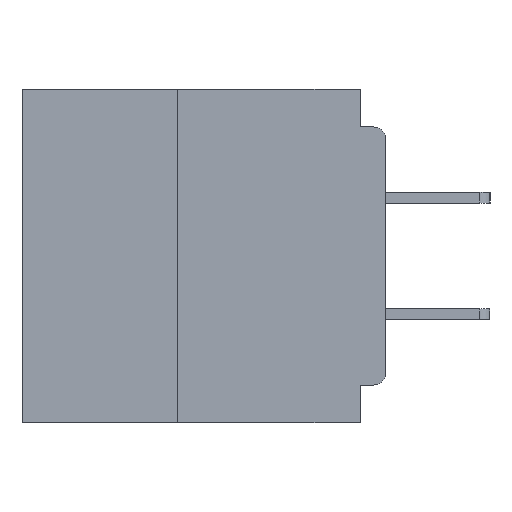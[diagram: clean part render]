
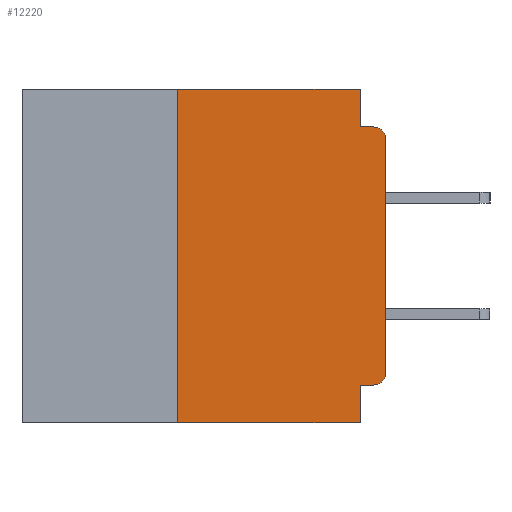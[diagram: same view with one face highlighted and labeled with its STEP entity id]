
A CAD part, left-side view. The second image highlights one B-rep face of the part: STEP entity #12220.
In plain terms, the highlighted planar face has unit normal (-1, 0, 0).
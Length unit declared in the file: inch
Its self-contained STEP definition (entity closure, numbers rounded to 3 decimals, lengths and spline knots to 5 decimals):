
#290 = EDGE_CURVE ( 'NONE', #17240, #39688, #41351, .T. ) ;
#2106 = VECTOR ( 'NONE', #35604, 39.37008 ) ;
#2273 = AXIS2_PLACEMENT_3D ( 'NONE', #43329, #23393, #3260 ) ;
#3179 = LINE ( 'NONE', #18745, #2106 ) ;
#3260 = DIRECTION ( 'NONE',  ( 0., 0., -1. ) ) ;
#4384 = ORIENTED_EDGE ( 'NONE', *, *, #42778, .F. ) ;
#4550 = EDGE_CURVE ( 'NONE', #42149, #12079, #9483, .T. ) ;
#6337 = VECTOR ( 'NONE', #36589, 39.37008 ) ;
#6389 = DIRECTION ( 'NONE',  ( 0., 0., -1. ) ) ;
#6859 = CARTESIAN_POINT ( 'NONE',  ( 0., 0., -0.06 ) ) ;
#7422 = ORIENTED_EDGE ( 'NONE', *, *, #15491, .F. ) ;
#8079 = LINE ( 'NONE', #9819, #24924 ) ;
#9199 = CIRCLE ( 'NONE', #23481, 0.015 ) ;
#9483 = LINE ( 'NONE', #37488, #17401 ) ;
#9774 = CARTESIAN_POINT ( 'NONE',  ( 0., 0.031, -0.4 ) ) ;
#9819 = CARTESIAN_POINT ( 'NONE',  ( 0., 0.031, 0. ) ) ;
#10661 = DIRECTION ( 'NONE',  ( 0., 1., 0. ) ) ;
#11162 = LINE ( 'NONE', #37138, #19002 ) ;
#11334 = PLANE ( 'NONE',  #36453 ) ;
#11867 = CARTESIAN_POINT ( 'NONE',  ( 0., 0., -0.34 ) ) ;
#12079 = VERTEX_POINT ( 'NONE', #40723 ) ;
#12220 = ADVANCED_FACE ( 'NONE', ( #42711 ), #11334, .F. ) ;
#13265 = CARTESIAN_POINT ( 'NONE',  ( 0., 0.015, -0.34 ) ) ;
#14462 = VECTOR ( 'NONE', #22229, 39.37008 ) ;
#14726 = DIRECTION ( 'NONE',  ( 1., 0., 0. ) ) ;
#15491 = EDGE_CURVE ( 'NONE', #17240, #26079, #11162, .T. ) ;
#15524 = CARTESIAN_POINT ( 'NONE',  ( 0., 0., 0. ) ) ;
#16160 = ORIENTED_EDGE ( 'NONE', *, *, #29228, .T. ) ;
#16396 = EDGE_CURVE ( 'NONE', #26079, #41114, #3179, .T. ) ;
#16649 = DIRECTION ( 'NONE',  ( 0., 0., -1. ) ) ;
#16746 = DIRECTION ( 'NONE',  ( 0., 0., -1. ) ) ;
#17018 = VERTEX_POINT ( 'NONE', #39463 ) ;
#17073 = DIRECTION ( 'NONE',  ( 0., 0., 1. ) ) ;
#17240 = VERTEX_POINT ( 'NONE', #27374 ) ;
#17401 = VECTOR ( 'NONE', #10661, 39.37008 ) ;
#18265 = ORIENTED_EDGE ( 'NONE', *, *, #35848, .T. ) ;
#18745 = CARTESIAN_POINT ( 'NONE',  ( 0., 0.437, 0. ) ) ;
#18962 = ORIENTED_EDGE ( 'NONE', *, *, #16396, .F. ) ;
#19002 = VECTOR ( 'NONE', #17073, 39.37008 ) ;
#19512 = ORIENTED_EDGE ( 'NONE', *, *, #290, .T. ) ;
#19656 = CARTESIAN_POINT ( 'NONE',  ( 0., 0.015, -0.355 ) ) ;
#20875 = CARTESIAN_POINT ( 'NONE',  ( 0., 0.25, 0. ) ) ;
#21302 = CARTESIAN_POINT ( 'NONE',  ( 0., 0.437, 0. ) ) ;
#22229 = DIRECTION ( 'NONE',  ( 0., 0., 1. ) ) ;
#23393 = DIRECTION ( 'NONE',  ( -1., 0., 0. ) ) ;
#23481 = AXIS2_PLACEMENT_3D ( 'NONE', #13265, #36714, #16649 ) ;
#24924 = VECTOR ( 'NONE', #16746, 39.37008 ) ;
#25423 = LINE ( 'NONE', #9774, #42065 ) ;
#25580 = DIRECTION ( 'NONE',  ( 0., -1., 0. ) ) ;
#25952 = CARTESIAN_POINT ( 'NONE',  ( 0., 0.015, -0.045 ) ) ;
#25984 = ORIENTED_EDGE ( 'NONE', *, *, #27196, .F. ) ;
#26079 = VERTEX_POINT ( 'NONE', #20875 ) ;
#26563 = CARTESIAN_POINT ( 'NONE',  ( 0., 0.437, -0.4 ) ) ;
#27087 = VERTEX_POINT ( 'NONE', #25952 ) ;
#27196 = EDGE_CURVE ( 'NONE', #12079, #39688, #25423, .T. ) ;
#27374 = CARTESIAN_POINT ( 'NONE',  ( 0., 0.25, -0.4 ) ) ;
#28415 = VERTEX_POINT ( 'NONE', #11867 ) ;
#29228 = EDGE_CURVE ( 'NONE', #41108, #27087, #41705, .T. ) ;
#30398 = CARTESIAN_POINT ( 'NONE',  ( 0., 0.031, 0. ) ) ;
#30609 = EDGE_CURVE ( 'NONE', #41114, #17018, #8079, .T. ) ;
#32571 = VECTOR ( 'NONE', #25580, 39.37008 ) ;
#32693 = CARTESIAN_POINT ( 'NONE',  ( 0., 0.031, -0.4 ) ) ;
#33252 = CARTESIAN_POINT ( 'NONE',  ( 0., 0., -0.045 ) ) ;
#33691 = ORIENTED_EDGE ( 'NONE', *, *, #30609, .F. ) ;
#35604 = DIRECTION ( 'NONE',  ( 0., -1., 0. ) ) ;
#35848 = EDGE_CURVE ( 'NONE', #28415, #41108, #41112, .T. ) ;
#36453 = AXIS2_PLACEMENT_3D ( 'NONE', #21302, #14726, #38153 ) ;
#36589 = DIRECTION ( 'NONE',  ( 0., -1., 0. ) ) ;
#36714 = DIRECTION ( 'NONE',  ( -1., 0., 0. ) ) ;
#37138 = CARTESIAN_POINT ( 'NONE',  ( 0., 0.25, -0.4 ) ) ;
#37488 = CARTESIAN_POINT ( 'NONE',  ( 0., 0., -0.355 ) ) ;
#38153 = DIRECTION ( 'NONE',  ( 0., 0., -1. ) ) ;
#39257 = ORIENTED_EDGE ( 'NONE', *, *, #40376, .T. ) ;
#39463 = CARTESIAN_POINT ( 'NONE',  ( 0., 0.031, -0.045 ) ) ;
#39688 = VERTEX_POINT ( 'NONE', #32693 ) ;
#40376 = EDGE_CURVE ( 'NONE', #42149, #28415, #9199, .T. ) ;
#40723 = CARTESIAN_POINT ( 'NONE',  ( 0., 0.031, -0.355 ) ) ;
#41108 = VERTEX_POINT ( 'NONE', #6859 ) ;
#41112 = LINE ( 'NONE', #15524, #14462 ) ;
#41114 = VERTEX_POINT ( 'NONE', #30398 ) ;
#41351 = LINE ( 'NONE', #26563, #32571 ) ;
#41705 = CIRCLE ( 'NONE', #2273, 0.015 ) ;
#41934 = LINE ( 'NONE', #33252, #6337 ) ;
#42065 = VECTOR ( 'NONE', #6389, 39.37008 ) ;
#42073 = EDGE_LOOP ( 'NONE', ( #18265, #16160, #4384, #33691, #18962, #7422, #19512, #25984, #42876, #39257 ) ) ;
#42149 = VERTEX_POINT ( 'NONE', #19656 ) ;
#42711 = FACE_OUTER_BOUND ( 'NONE', #42073, .T. ) ;
#42778 = EDGE_CURVE ( 'NONE', #17018, #27087, #41934, .T. ) ;
#42876 = ORIENTED_EDGE ( 'NONE', *, *, #4550, .F. ) ;
#43329 = CARTESIAN_POINT ( 'NONE',  ( 0., 0.015, -0.06 ) ) ;
